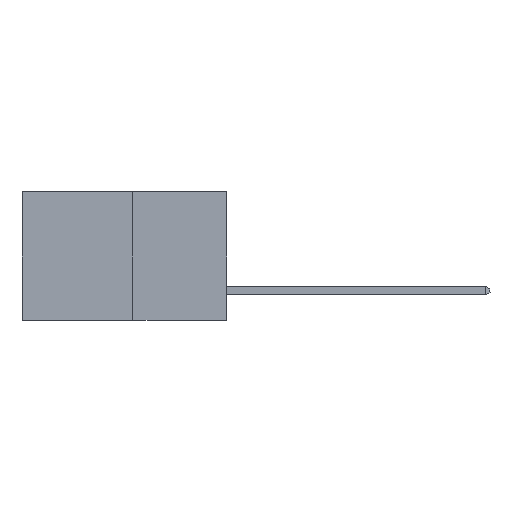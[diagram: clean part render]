
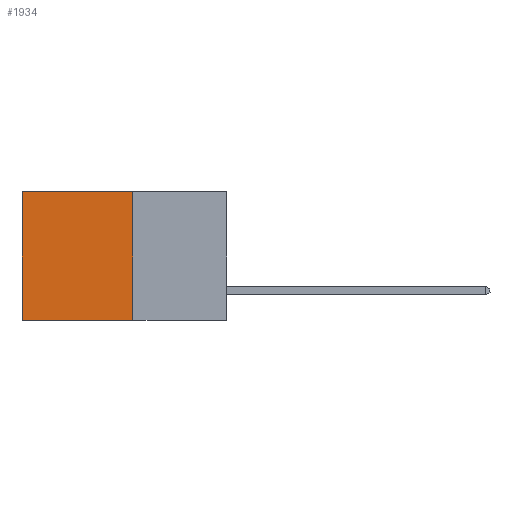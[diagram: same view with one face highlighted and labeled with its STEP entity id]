
A CAD part, left-side view. The second image highlights one B-rep face of the part: STEP entity #1934.
In plain terms, the highlighted planar face has unit normal (-1, 0, 0).
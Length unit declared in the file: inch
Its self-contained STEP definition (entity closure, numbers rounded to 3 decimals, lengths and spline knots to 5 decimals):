
#737 = CARTESIAN_POINT ( 'NONE',  ( 0.277, 0.27, 0. ) ) ;
#1038 = ORIENTED_EDGE ( 'NONE', *, *, #2840, .F. ) ;
#1238 = VERTEX_POINT ( 'NONE', #4191 ) ;
#1284 = DIRECTION ( 'NONE',  ( 0., 1., 0. ) ) ;
#1338 = EDGE_CURVE ( 'NONE', #11353, #6312, #11314, .T. ) ;
#1569 = EDGE_CURVE ( 'NONE', #11353, #5923, #8936, .T. ) ;
#1716 = DIRECTION ( 'NONE',  ( 0., 1., 0. ) ) ;
#1934 = ADVANCED_FACE ( 'NONE', ( #12604 ), #6330, .F. ) ;
#1975 = CARTESIAN_POINT ( 'NONE',  ( 0.277, 0.59, -0.37 ) ) ;
#1983 = ORIENTED_EDGE ( 'NONE', *, *, #5089, .T. ) ;
#2840 = EDGE_CURVE ( 'NONE', #5923, #1238, #8760, .T. ) ;
#3033 = DIRECTION ( 'NONE',  ( 0., 0., -1. ) ) ;
#4191 = CARTESIAN_POINT ( 'NONE',  ( 0.277, 0.59, -0.37 ) ) ;
#4224 = EDGE_LOOP ( 'NONE', ( #1983, #1038, #7282, #5261 ) ) ;
#4242 = DIRECTION ( 'NONE',  ( 1., 0., 0. ) ) ;
#4294 = DIRECTION ( 'NONE',  ( 0., 0., -1. ) ) ;
#4448 = CARTESIAN_POINT ( 'NONE',  ( 0.277, 0.27, -0.37 ) ) ;
#4472 = DIRECTION ( 'NONE',  ( 0., 0., -1. ) ) ;
#4670 = CARTESIAN_POINT ( 'NONE',  ( 0.277, 0.27, -0.37 ) ) ;
#5047 = CARTESIAN_POINT ( 'NONE',  ( 0.277, 0.27, -0.37 ) ) ;
#5089 = EDGE_CURVE ( 'NONE', #6312, #1238, #6311, .T. ) ;
#5261 = ORIENTED_EDGE ( 'NONE', *, *, #1338, .T. ) ;
#5923 = VERTEX_POINT ( 'NONE', #4670 ) ;
#6311 = LINE ( 'NONE', #1975, #7928 ) ;
#6312 = VERTEX_POINT ( 'NONE', #10962 ) ;
#6330 = PLANE ( 'NONE',  #8399 ) ;
#7139 = CARTESIAN_POINT ( 'NONE',  ( 0.277, 0.27, -0.37 ) ) ;
#7282 = ORIENTED_EDGE ( 'NONE', *, *, #1569, .F. ) ;
#7928 = VECTOR ( 'NONE', #3033, 39.37008 ) ;
#8399 = AXIS2_PLACEMENT_3D ( 'NONE', #7139, #4242, #4294 ) ;
#8631 = VECTOR ( 'NONE', #4472, 39.37008 ) ;
#8760 = LINE ( 'NONE', #5047, #10087 ) ;
#8936 = LINE ( 'NONE', #4448, #8631 ) ;
#10087 = VECTOR ( 'NONE', #1716, 39.37008 ) ;
#10695 = CARTESIAN_POINT ( 'NONE',  ( 0.277, 0.27, 0. ) ) ;
#10962 = CARTESIAN_POINT ( 'NONE',  ( 0.277, 0.59, 0. ) ) ;
#11010 = VECTOR ( 'NONE', #1284, 39.37008 ) ;
#11314 = LINE ( 'NONE', #737, #11010 ) ;
#11353 = VERTEX_POINT ( 'NONE', #10695 ) ;
#12604 = FACE_OUTER_BOUND ( 'NONE', #4224, .T. ) ;
